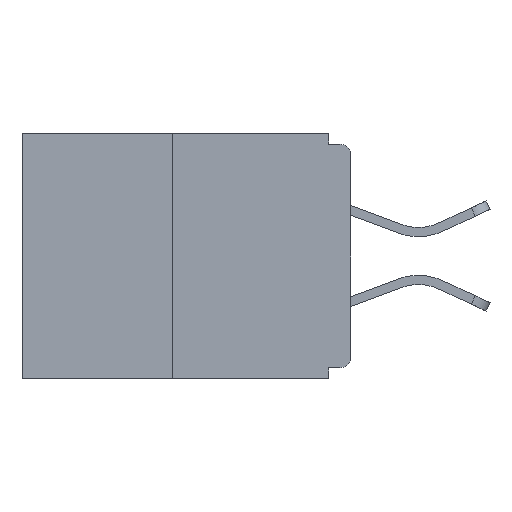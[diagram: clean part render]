
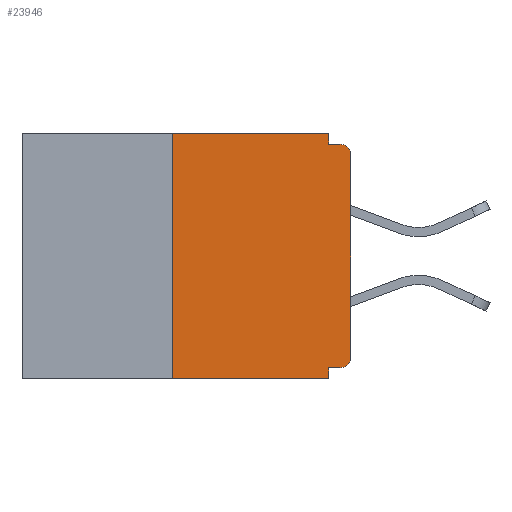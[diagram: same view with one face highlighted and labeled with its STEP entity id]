
A CAD part, left-side view. The second image highlights one B-rep face of the part: STEP entity #23946.
In plain terms, the highlighted planar face has unit normal (-1, 0, 0).
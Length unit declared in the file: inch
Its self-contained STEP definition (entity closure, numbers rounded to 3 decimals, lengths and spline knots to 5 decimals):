
#6 = EDGE_CURVE ( 'NONE', #5587, #7027, #8438, .T. ) ;
#136 = LINE ( 'NONE', #197, #13293 ) ;
#197 = CARTESIAN_POINT ( 'NONE',  ( 0., 0.25, 0. ) ) ;
#414 = ORIENTED_EDGE ( 'NONE', *, *, #23290, .F. ) ;
#885 = AXIS2_PLACEMENT_3D ( 'NONE', #24042, #19825, #6582 ) ;
#1135 = CARTESIAN_POINT ( 'NONE',  ( 0., 0., -0.015 ) ) ;
#1352 = CARTESIAN_POINT ( 'NONE',  ( 0., 0.031, -0.328 ) ) ;
#1439 = CARTESIAN_POINT ( 'NONE',  ( 0., 0.031, -0.343 ) ) ;
#1618 = LINE ( 'NONE', #21781, #22680 ) ;
#2146 = ORIENTED_EDGE ( 'NONE', *, *, #12152, .T. ) ;
#2429 = VECTOR ( 'NONE', #17300, 39.37008 ) ;
#3360 = VECTOR ( 'NONE', #7493, 39.37008 ) ;
#3863 = ORIENTED_EDGE ( 'NONE', *, *, #16491, .F. ) ;
#3944 = ORIENTED_EDGE ( 'NONE', *, *, #8166, .F. ) ;
#4561 = CARTESIAN_POINT ( 'NONE',  ( 0., 0.031, -0.015 ) ) ;
#5587 = VERTEX_POINT ( 'NONE', #10673 ) ;
#6450 = EDGE_CURVE ( 'NONE', #20059, #19472, #15117, .T. ) ;
#6582 = DIRECTION ( 'NONE',  ( 0., 0., -1. ) ) ;
#6722 = LINE ( 'NONE', #1439, #26393 ) ;
#6874 = DIRECTION ( 'NONE',  ( -1., 0., 0. ) ) ;
#7027 = VERTEX_POINT ( 'NONE', #28202 ) ;
#7493 = DIRECTION ( 'NONE',  ( 0., -1., 0. ) ) ;
#8067 = VECTOR ( 'NONE', #25155, 39.37008 ) ;
#8166 = EDGE_CURVE ( 'NONE', #20059, #5587, #136, .T. ) ;
#8284 = LINE ( 'NONE', #15277, #2429 ) ;
#8432 = CARTESIAN_POINT ( 'NONE',  ( 0., 0.46, -0.343 ) ) ;
#8438 = LINE ( 'NONE', #11572, #18806 ) ;
#8804 = ORIENTED_EDGE ( 'NONE', *, *, #25048, .F. ) ;
#9083 = EDGE_LOOP ( 'NONE', ( #20209, #3944, #22295, #8804, #414, #13190, #2146, #28389, #3863, #9973 ) ) ;
#9492 = VERTEX_POINT ( 'NONE', #10944 ) ;
#9765 = CARTESIAN_POINT ( 'NONE',  ( 0., 0., 0. ) ) ;
#9973 = ORIENTED_EDGE ( 'NONE', *, *, #18522, .F. ) ;
#10673 = CARTESIAN_POINT ( 'NONE',  ( 0., 0.25, 0. ) ) ;
#10944 = CARTESIAN_POINT ( 'NONE',  ( 0., 0., -0.03 ) ) ;
#11144 = PLANE ( 'NONE',  #885 ) ;
#11572 = CARTESIAN_POINT ( 'NONE',  ( 0., 0.46, 0. ) ) ;
#12152 = EDGE_CURVE ( 'NONE', #15250, #9492, #13956, .T. ) ;
#12621 = DIRECTION ( 'NONE',  ( 0., -1., 0. ) ) ;
#12693 = AXIS2_PLACEMENT_3D ( 'NONE', #21925, #6874, #24226 ) ;
#12706 = DIRECTION ( 'NONE',  ( 0., 0., -1. ) ) ;
#13037 = VECTOR ( 'NONE', #12621, 39.37008 ) ;
#13190 = ORIENTED_EDGE ( 'NONE', *, *, #19233, .T. ) ;
#13196 = AXIS2_PLACEMENT_3D ( 'NONE', #17230, #28447, #12706 ) ;
#13293 = VECTOR ( 'NONE', #26438, 39.37008 ) ;
#13956 = LINE ( 'NONE', #9765, #8067 ) ;
#15117 = LINE ( 'NONE', #8432, #13037 ) ;
#15250 = VERTEX_POINT ( 'NONE', #17432 ) ;
#15277 = CARTESIAN_POINT ( 'NONE',  ( 0., 0.031, 0. ) ) ;
#16086 = DIRECTION ( 'NONE',  ( 0., -1., 0. ) ) ;
#16111 = VERTEX_POINT ( 'NONE', #19827 ) ;
#16219 = CIRCLE ( 'NONE', #13196, 0.015 ) ;
#16491 = EDGE_CURVE ( 'NONE', #23982, #19209, #18882, .T. ) ;
#17230 = CARTESIAN_POINT ( 'NONE',  ( 0., 0.015, -0.313 ) ) ;
#17300 = DIRECTION ( 'NONE',  ( 0., 0., -1. ) ) ;
#17432 = CARTESIAN_POINT ( 'NONE',  ( 0., 0., -0.313 ) ) ;
#17778 = CIRCLE ( 'NONE', #12693, 0.015 ) ;
#18522 = EDGE_CURVE ( 'NONE', #7027, #23982, #8284, .T. ) ;
#18806 = VECTOR ( 'NONE', #16086, 39.37008 ) ;
#18882 = LINE ( 'NONE', #1135, #3360 ) ;
#18891 = DIRECTION ( 'NONE',  ( 0., 0., -1. ) ) ;
#19062 = CARTESIAN_POINT ( 'NONE',  ( 0., 0.015, -0.015 ) ) ;
#19209 = VERTEX_POINT ( 'NONE', #19062 ) ;
#19233 = EDGE_CURVE ( 'NONE', #16111, #15250, #16219, .T. ) ;
#19472 = VERTEX_POINT ( 'NONE', #19836 ) ;
#19825 = DIRECTION ( 'NONE',  ( 1., 0., 0. ) ) ;
#19827 = CARTESIAN_POINT ( 'NONE',  ( 0., 0.015, -0.328 ) ) ;
#19836 = CARTESIAN_POINT ( 'NONE',  ( 0., 0.031, -0.343 ) ) ;
#19949 = DIRECTION ( 'NONE',  ( 0., 1., 0. ) ) ;
#20059 = VERTEX_POINT ( 'NONE', #25536 ) ;
#20209 = ORIENTED_EDGE ( 'NONE', *, *, #6, .F. ) ;
#21781 = CARTESIAN_POINT ( 'NONE',  ( 0., 0., -0.328 ) ) ;
#21925 = CARTESIAN_POINT ( 'NONE',  ( 0., 0.015, -0.03 ) ) ;
#22295 = ORIENTED_EDGE ( 'NONE', *, *, #6450, .T. ) ;
#22376 = EDGE_CURVE ( 'NONE', #9492, #19209, #17778, .T. ) ;
#22680 = VECTOR ( 'NONE', #19949, 39.37008 ) ;
#23290 = EDGE_CURVE ( 'NONE', #16111, #28220, #1618, .T. ) ;
#23946 = ADVANCED_FACE ( 'NONE', ( #27455 ), #11144, .F. ) ;
#23982 = VERTEX_POINT ( 'NONE', #4561 ) ;
#24042 = CARTESIAN_POINT ( 'NONE',  ( 0., 0.46, 0. ) ) ;
#24226 = DIRECTION ( 'NONE',  ( 0., 0., -1. ) ) ;
#25048 = EDGE_CURVE ( 'NONE', #28220, #19472, #6722, .T. ) ;
#25155 = DIRECTION ( 'NONE',  ( 0., 0., 1. ) ) ;
#25536 = CARTESIAN_POINT ( 'NONE',  ( 0., 0.25, -0.343 ) ) ;
#26393 = VECTOR ( 'NONE', #18891, 39.37008 ) ;
#26438 = DIRECTION ( 'NONE',  ( 0., 0., 1. ) ) ;
#27455 = FACE_OUTER_BOUND ( 'NONE', #9083, .T. ) ;
#28202 = CARTESIAN_POINT ( 'NONE',  ( 0., 0.031, 0. ) ) ;
#28220 = VERTEX_POINT ( 'NONE', #1352 ) ;
#28389 = ORIENTED_EDGE ( 'NONE', *, *, #22376, .T. ) ;
#28447 = DIRECTION ( 'NONE',  ( -1., 0., 0. ) ) ;
